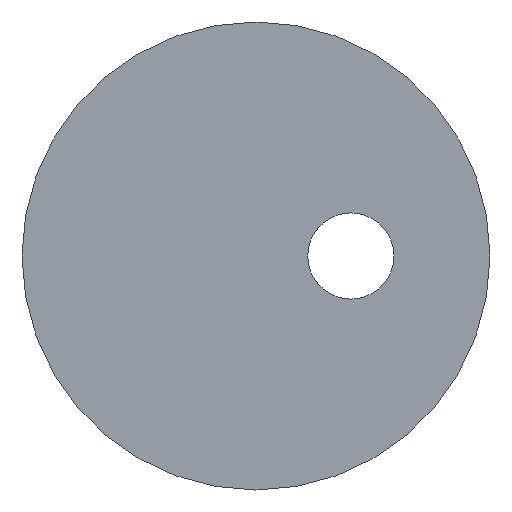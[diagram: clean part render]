
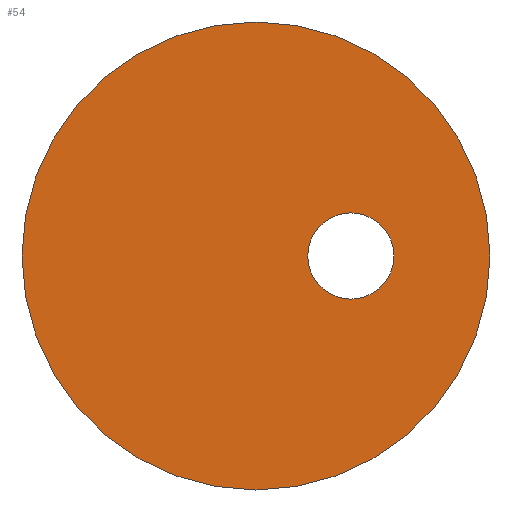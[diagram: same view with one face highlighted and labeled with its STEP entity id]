
A CAD part, left-side view. The second image highlights one B-rep face of the part: STEP entity #54.
In plain terms, the highlighted planar face has unit normal (-1, 0, 0).
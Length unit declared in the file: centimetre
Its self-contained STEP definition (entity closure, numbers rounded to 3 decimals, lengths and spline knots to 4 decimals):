
#13=PLANE($,#63);
#16=FACE_BOUND($,#26,.T.);
#20=FACE_OUTER_BOUND($,#25,.T.);
#25=EDGE_LOOP($,(#45));
#26=EDGE_LOOP($,(#46));
#32=CIRCLE($,#62,0.95);
#33=CIRCLE($,#64,0.175);
#36=VERTEX_POINT($,#90);
#37=VERTEX_POINT($,#93);
#40=EDGE_CURVE($,#36,#36,#32,.F.);
#41=EDGE_CURVE($,#37,#37,#33,.T.);
#45=ORIENTED_EDGE($,*,*,#40,.F.);
#46=ORIENTED_EDGE($,*,*,#41,.F.);
#54=ADVANCED_FACE($,(#20,#16),#13,.T.);
#62=AXIS2_PLACEMENT_3D($,#91,#74,#75);
#63=AXIS2_PLACEMENT_3D($,#92,#76,#77);
#64=AXIS2_PLACEMENT_3D($,#94,#78,#79);
#74=DIRECTION('center_axis',(-1.,0.,0.));
#75=DIRECTION('ref_axis',(0.,0.,
1.));
#76=DIRECTION('center_axis',(-1.,0.,0.));
#77=DIRECTION('ref_axis',(0.,0.,-1.));
#78=DIRECTION('center_axis',(-1.,0.,0.));
#79=DIRECTION('ref_axis',(0.,0.,
1.));
#90=CARTESIAN_POINT('',(-6.64,2.7397,-0.8819));
#91=CARTESIAN_POINT('Origin',(-6.64,2.7397,0.0681));
#92=CARTESIAN_POINT('Origin',(-6.64,2.7397,1.0181));
#93=CARTESIAN_POINT('',(-6.64,2.3547,-0.1069));
#94=CARTESIAN_POINT('Origin',(-6.64,2.3547,0.0681));
